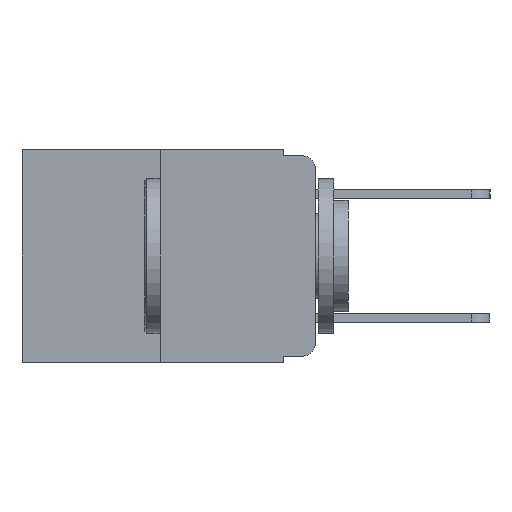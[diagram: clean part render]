
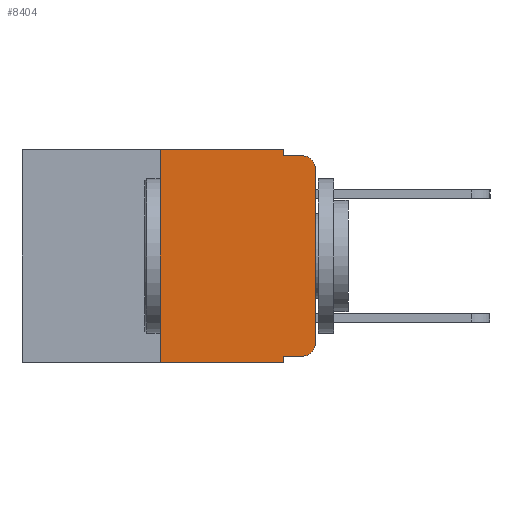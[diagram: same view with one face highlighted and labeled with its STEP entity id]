
A CAD part, left-side view. The second image highlights one B-rep face of the part: STEP entity #8404.
In plain terms, the highlighted planar face has unit normal (-1, 0, 0).
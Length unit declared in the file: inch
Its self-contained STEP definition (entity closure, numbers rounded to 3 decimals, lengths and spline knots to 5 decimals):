
#119 = VERTEX_POINT ( 'NONE', #10000 ) ;
#191 = EDGE_CURVE ( 'NONE', #4502, #7558, #5999, .T. ) ;
#336 = DIRECTION ( 'NONE',  ( 0., -1., 0. ) ) ;
#545 = DIRECTION ( 'NONE',  ( 0., 0., -1. ) ) ;
#852 = DIRECTION ( 'NONE',  ( 0., -1., 0. ) ) ;
#1249 = AXIS2_PLACEMENT_3D ( 'NONE', #4314, #10748, #5219 ) ;
#1390 = ORIENTED_EDGE ( 'NONE', *, *, #3156, .T. ) ;
#1474 = CARTESIAN_POINT ( 'NONE',  ( 0., 0.051, -0.01 ) ) ;
#1483 = AXIS2_PLACEMENT_3D ( 'NONE', #9636, #4139, #10575 ) ;
#1792 = AXIS2_PLACEMENT_3D ( 'NONE', #3502, #5361, #11793 ) ;
#1925 = LINE ( 'NONE', #3648, #6536 ) ;
#2002 = CARTESIAN_POINT ( 'NONE',  ( 0., 0., -0.313 ) ) ;
#2342 = CARTESIAN_POINT ( 'NONE',  ( 0., 0.051, 0. ) ) ;
#2768 = VECTOR ( 'NONE', #336, 39.37008 ) ;
#2981 = ORIENTED_EDGE ( 'NONE', *, *, #9557, .T. ) ;
#3005 = EDGE_CURVE ( 'NONE', #6040, #3755, #3350, .T. ) ;
#3156 = EDGE_CURVE ( 'NONE', #3755, #7943, #1925, .T. ) ;
#3159 = VERTEX_POINT ( 'NONE', #8213 ) ;
#3350 = CIRCLE ( 'NONE', #1249, 0.02 ) ;
#3459 = PLANE ( 'NONE',  #1792 ) ;
#3502 = CARTESIAN_POINT ( 'NONE',  ( 0., 0.473, 0. ) ) ;
#3557 = DIRECTION ( 'NONE',  ( 0., 0., 1. ) ) ;
#3648 = CARTESIAN_POINT ( 'NONE',  ( 0., 0., 0. ) ) ;
#3675 = ORIENTED_EDGE ( 'NONE', *, *, #7324, .T. ) ;
#3688 = ORIENTED_EDGE ( 'NONE', *, *, #9790, .F. ) ;
#3711 = DIRECTION ( 'NONE',  ( 0., 0., -1. ) ) ;
#3755 = VERTEX_POINT ( 'NONE', #2002 ) ;
#4023 = EDGE_CURVE ( 'NONE', #3159, #9072, #7641, .T. ) ;
#4139 = DIRECTION ( 'NONE',  ( -1., 0., 0. ) ) ;
#4314 = CARTESIAN_POINT ( 'NONE',  ( 0., 0.02, -0.313 ) ) ;
#4502 = VERTEX_POINT ( 'NONE', #7827 ) ;
#4856 = ORIENTED_EDGE ( 'NONE', *, *, #5244, .F. ) ;
#4932 = CARTESIAN_POINT ( 'NONE',  ( 0., 0.473, 0. ) ) ;
#5219 = DIRECTION ( 'NONE',  ( 0., 0., -1. ) ) ;
#5244 = EDGE_CURVE ( 'NONE', #9072, #119, #9764, .T. ) ;
#5361 = DIRECTION ( 'NONE',  ( 1., 0., 0. ) ) ;
#5364 = CARTESIAN_POINT ( 'NONE',  ( 0., 0.02, -0.333 ) ) ;
#5856 = ORIENTED_EDGE ( 'NONE', *, *, #3005, .T. ) ;
#5868 = ORIENTED_EDGE ( 'NONE', *, *, #10094, .F. ) ;
#5971 = LINE ( 'NONE', #10890, #10283 ) ;
#5999 = LINE ( 'NONE', #11805, #10010 ) ;
#6040 = VERTEX_POINT ( 'NONE', #5364 ) ;
#6168 = EDGE_LOOP ( 'NONE', ( #1390, #2981, #4856, #11901, #5868, #3688, #8700, #11886, #3675, #5856 ) ) ;
#6266 = VECTOR ( 'NONE', #852, 39.37008 ) ;
#6536 = VECTOR ( 'NONE', #10091, 39.37008 ) ;
#6562 = LINE ( 'NONE', #10990, #6266 ) ;
#7072 = VECTOR ( 'NONE', #545, 39.37008 ) ;
#7276 = CARTESIAN_POINT ( 'NONE',  ( 0., 0.051, -0.333 ) ) ;
#7308 = VERTEX_POINT ( 'NONE', #7276 ) ;
#7316 = VECTOR ( 'NONE', #8819, 39.37008 ) ;
#7324 = EDGE_CURVE ( 'NONE', #7308, #6040, #6562, .T. ) ;
#7558 = VERTEX_POINT ( 'NONE', #10418 ) ;
#7641 = LINE ( 'NONE', #2342, #7072 ) ;
#7827 = CARTESIAN_POINT ( 'NONE',  ( 0., 0.25, -0.343 ) ) ;
#7943 = VERTEX_POINT ( 'NONE', #8250 ) ;
#8213 = CARTESIAN_POINT ( 'NONE',  ( 0., 0.051, 0. ) ) ;
#8250 = CARTESIAN_POINT ( 'NONE',  ( 0., 0., -0.03 ) ) ;
#8284 = CARTESIAN_POINT ( 'NONE',  ( 0., 0.051, 0. ) ) ;
#8404 = ADVANCED_FACE ( 'NONE', ( #10604 ), #3459, .F. ) ;
#8503 = VERTEX_POINT ( 'NONE', #10074 ) ;
#8545 = EDGE_CURVE ( 'NONE', #7308, #7558, #9138, .T. ) ;
#8700 = ORIENTED_EDGE ( 'NONE', *, *, #191, .T. ) ;
#8819 = DIRECTION ( 'NONE',  ( 0., -1., 0. ) ) ;
#9072 = VERTEX_POINT ( 'NONE', #10062 ) ;
#9138 = LINE ( 'NONE', #8284, #11600 ) ;
#9269 = DIRECTION ( 'NONE',  ( 0., -1., 0. ) ) ;
#9536 = LINE ( 'NONE', #4932, #2768 ) ;
#9557 = EDGE_CURVE ( 'NONE', #7943, #119, #10720, .T. ) ;
#9636 = CARTESIAN_POINT ( 'NONE',  ( 0., 0.02, -0.03 ) ) ;
#9764 = LINE ( 'NONE', #1474, #7316 ) ;
#9790 = EDGE_CURVE ( 'NONE', #4502, #8503, #5971, .T. ) ;
#10000 = CARTESIAN_POINT ( 'NONE',  ( 0., 0.02, -0.01 ) ) ;
#10010 = VECTOR ( 'NONE', #9269, 39.37008 ) ;
#10062 = CARTESIAN_POINT ( 'NONE',  ( 0., 0.051, -0.01 ) ) ;
#10074 = CARTESIAN_POINT ( 'NONE',  ( 0., 0.25, 0. ) ) ;
#10091 = DIRECTION ( 'NONE',  ( 0., 0., 1. ) ) ;
#10094 = EDGE_CURVE ( 'NONE', #8503, #3159, #9536, .T. ) ;
#10283 = VECTOR ( 'NONE', #3557, 39.37008 ) ;
#10418 = CARTESIAN_POINT ( 'NONE',  ( 0., 0.051, -0.343 ) ) ;
#10575 = DIRECTION ( 'NONE',  ( 0., 0., -1. ) ) ;
#10604 = FACE_OUTER_BOUND ( 'NONE', #6168, .T. ) ;
#10720 = CIRCLE ( 'NONE', #1483, 0.02 ) ;
#10748 = DIRECTION ( 'NONE',  ( -1., 0., 0. ) ) ;
#10890 = CARTESIAN_POINT ( 'NONE',  ( 0., 0.25, 0. ) ) ;
#10990 = CARTESIAN_POINT ( 'NONE',  ( 0., 0.051, -0.333 ) ) ;
#11600 = VECTOR ( 'NONE', #3711, 39.37008 ) ;
#11793 = DIRECTION ( 'NONE',  ( 0., 0., -1. ) ) ;
#11805 = CARTESIAN_POINT ( 'NONE',  ( 0., 0.473, -0.343 ) ) ;
#11886 = ORIENTED_EDGE ( 'NONE', *, *, #8545, .F. ) ;
#11901 = ORIENTED_EDGE ( 'NONE', *, *, #4023, .F. ) ;
